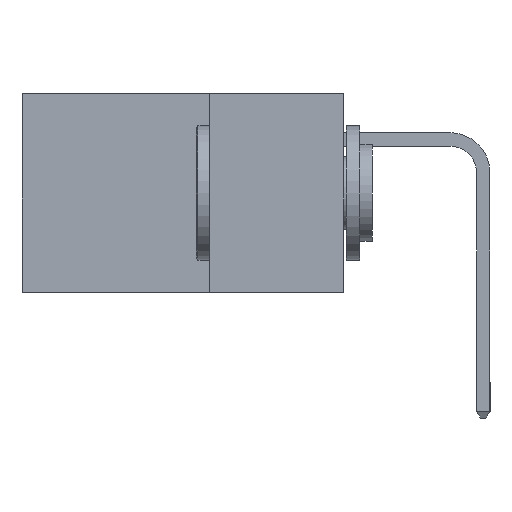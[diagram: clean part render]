
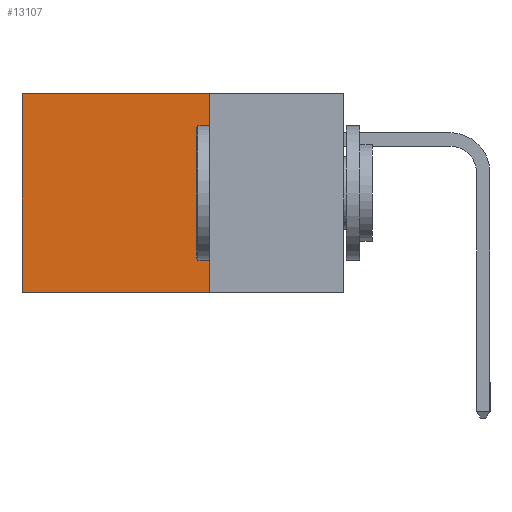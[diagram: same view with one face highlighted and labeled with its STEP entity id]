
A CAD part, left-side view. The second image highlights one B-rep face of the part: STEP entity #13107.
In plain terms, the highlighted planar face has unit normal (-1, 0, 0).
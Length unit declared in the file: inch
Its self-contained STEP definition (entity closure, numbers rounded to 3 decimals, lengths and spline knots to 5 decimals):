
#229 = ORIENTED_EDGE ( 'NONE', *, *, #10441, .F. ) ;
#266 = ORIENTED_EDGE ( 'NONE', *, *, #2852, .T. ) ;
#776 = LINE ( 'NONE', #8661, #10419 ) ;
#1278 = CARTESIAN_POINT ( 'NONE',  ( 0.298, 0.6, 0. ) ) ;
#1696 = DIRECTION ( 'NONE',  ( 0., 1., 0. ) ) ;
#1745 = VECTOR ( 'NONE', #4867, 39.37008 ) ;
#2689 = VERTEX_POINT ( 'NONE', #9529 ) ;
#2818 = FACE_OUTER_BOUND ( 'NONE', #4196, .T. ) ;
#2852 = EDGE_CURVE ( 'NONE', #6848, #2689, #7095, .T. ) ;
#3700 = CARTESIAN_POINT ( 'NONE',  ( 0.298, 0.25, 0. ) ) ;
#4196 = EDGE_LOOP ( 'NONE', ( #266, #229, #6860, #5126 ) ) ;
#4784 = CARTESIAN_POINT ( 'NONE',  ( 0.298, 0.25, 0. ) ) ;
#4867 = DIRECTION ( 'NONE',  ( 0., 0., -1. ) ) ;
#5126 = ORIENTED_EDGE ( 'NONE', *, *, #13346, .T. ) ;
#5969 = DIRECTION ( 'NONE',  ( 0., 1., 0. ) ) ;
#6199 = AXIS2_PLACEMENT_3D ( 'NONE', #7803, #6689, #14491 ) ;
#6689 = DIRECTION ( 'NONE',  ( 1., 0., 0. ) ) ;
#6848 = VERTEX_POINT ( 'NONE', #8716 ) ;
#6860 = ORIENTED_EDGE ( 'NONE', *, *, #7257, .F. ) ;
#7095 = LINE ( 'NONE', #1278, #10151 ) ;
#7257 = EDGE_CURVE ( 'NONE', #7935, #9317, #10967, .T. ) ;
#7719 = VECTOR ( 'NONE', #5969, 39.37008 ) ;
#7803 = CARTESIAN_POINT ( 'NONE',  ( 0.298, 0.25, 0. ) ) ;
#7935 = VERTEX_POINT ( 'NONE', #9425 ) ;
#8444 = LINE ( 'NONE', #4784, #7719 ) ;
#8661 = CARTESIAN_POINT ( 'NONE',  ( 0.298, 0.25, -0.37 ) ) ;
#8716 = CARTESIAN_POINT ( 'NONE',  ( 0.298, 0.6, 0. ) ) ;
#9317 = VERTEX_POINT ( 'NONE', #10010 ) ;
#9425 = CARTESIAN_POINT ( 'NONE',  ( 0.298, 0.25, 0. ) ) ;
#9529 = CARTESIAN_POINT ( 'NONE',  ( 0.298, 0.6, -0.37 ) ) ;
#10010 = CARTESIAN_POINT ( 'NONE',  ( 0.298, 0.25, -0.37 ) ) ;
#10151 = VECTOR ( 'NONE', #11157, 39.37008 ) ;
#10419 = VECTOR ( 'NONE', #1696, 39.37008 ) ;
#10441 = EDGE_CURVE ( 'NONE', #9317, #2689, #776, .T. ) ;
#10967 = LINE ( 'NONE', #3700, #1745 ) ;
#11157 = DIRECTION ( 'NONE',  ( 0., 0., -1. ) ) ;
#13107 = ADVANCED_FACE ( 'NONE', ( #2818 ), #13403, .F. ) ;
#13346 = EDGE_CURVE ( 'NONE', #7935, #6848, #8444, .T. ) ;
#13403 = PLANE ( 'NONE',  #6199 ) ;
#14491 = DIRECTION ( 'NONE',  ( 0., 0., -1. ) ) ;
